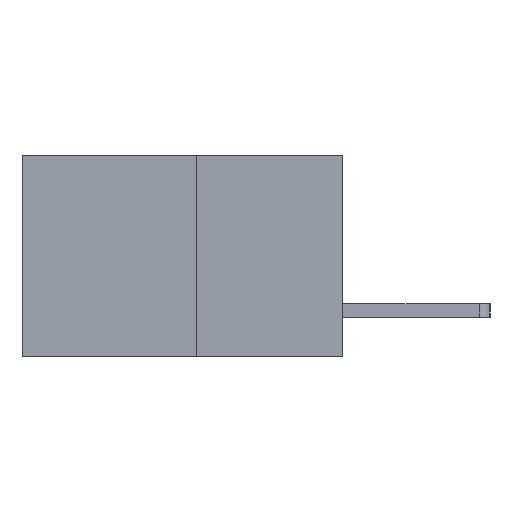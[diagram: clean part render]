
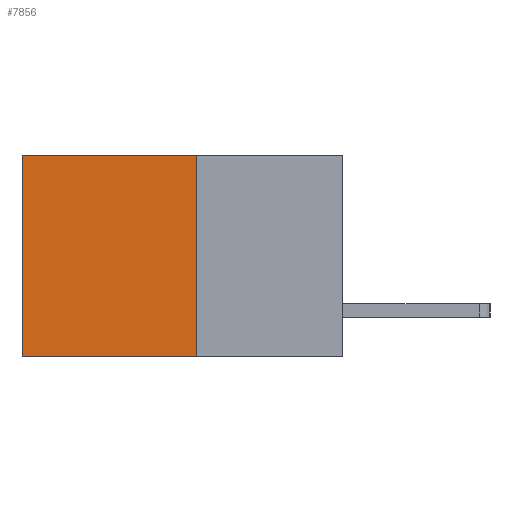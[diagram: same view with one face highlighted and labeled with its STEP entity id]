
A CAD part, left-side view. The second image highlights one B-rep face of the part: STEP entity #7856.
In plain terms, the highlighted planar face has unit normal (-1, 0, 0).
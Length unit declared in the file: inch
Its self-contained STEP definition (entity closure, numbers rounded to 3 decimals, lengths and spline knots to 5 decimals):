
#74 = VECTOR ( 'NONE', #4439, 39.37008 ) ;
#802 = ORIENTED_EDGE ( 'NONE', *, *, #6061, .F. ) ;
#894 = EDGE_LOOP ( 'NONE', ( #6322, #6533, #802, #6768 ) ) ;
#1026 = LINE ( 'NONE', #3760, #4326 ) ;
#1093 = EDGE_CURVE ( 'NONE', #3980, #3262, #3816, .T. ) ;
#1616 = FACE_OUTER_BOUND ( 'NONE', #894, .T. ) ;
#2114 = EDGE_CURVE ( 'NONE', #9240, #6102, #4119, .T. ) ;
#3003 = DIRECTION ( 'NONE',  ( 1., 0., 0. ) ) ;
#3241 = CARTESIAN_POINT ( 'NONE',  ( 0.277, 0.59, -0.37 ) ) ;
#3262 = VERTEX_POINT ( 'NONE', #6713 ) ;
#3725 = VECTOR ( 'NONE', #9517, 39.37008 ) ;
#3760 = CARTESIAN_POINT ( 'NONE',  ( 0.277, 0.27, -0.37 ) ) ;
#3816 = LINE ( 'NONE', #6958, #5563 ) ;
#3980 = VERTEX_POINT ( 'NONE', #6841 ) ;
#4119 = LINE ( 'NONE', #4182, #74 ) ;
#4182 = CARTESIAN_POINT ( 'NONE',  ( 0.277, 0.27, -0.37 ) ) ;
#4271 = AXIS2_PLACEMENT_3D ( 'NONE', #5838, #3003, #9236 ) ;
#4326 = VECTOR ( 'NONE', #6855, 39.37008 ) ;
#4439 = DIRECTION ( 'NONE',  ( 0., 1., 0. ) ) ;
#5562 = DIRECTION ( 'NONE',  ( 0., 1., 0. ) ) ;
#5563 = VECTOR ( 'NONE', #5562, 39.37008 ) ;
#5705 = LINE ( 'NONE', #8768, #3725 ) ;
#5838 = CARTESIAN_POINT ( 'NONE',  ( 0.277, 0.27, -0.37 ) ) ;
#6061 = EDGE_CURVE ( 'NONE', #3980, #9240, #1026, .T. ) ;
#6102 = VERTEX_POINT ( 'NONE', #3241 ) ;
#6322 = ORIENTED_EDGE ( 'NONE', *, *, #9192, .T. ) ;
#6533 = ORIENTED_EDGE ( 'NONE', *, *, #2114, .F. ) ;
#6713 = CARTESIAN_POINT ( 'NONE',  ( 0.277, 0.59, 0. ) ) ;
#6768 = ORIENTED_EDGE ( 'NONE', *, *, #1093, .T. ) ;
#6841 = CARTESIAN_POINT ( 'NONE',  ( 0.277, 0.27, 0. ) ) ;
#6855 = DIRECTION ( 'NONE',  ( 0., 0., -1. ) ) ;
#6958 = CARTESIAN_POINT ( 'NONE',  ( 0.277, 0.27, 0. ) ) ;
#7400 = CARTESIAN_POINT ( 'NONE',  ( 0.277, 0.27, -0.37 ) ) ;
#7802 = PLANE ( 'NONE',  #4271 ) ;
#7856 = ADVANCED_FACE ( 'NONE', ( #1616 ), #7802, .F. ) ;
#8768 = CARTESIAN_POINT ( 'NONE',  ( 0.277, 0.59, -0.37 ) ) ;
#9192 = EDGE_CURVE ( 'NONE', #3262, #6102, #5705, .T. ) ;
#9236 = DIRECTION ( 'NONE',  ( 0., 0., -1. ) ) ;
#9240 = VERTEX_POINT ( 'NONE', #7400 ) ;
#9517 = DIRECTION ( 'NONE',  ( 0., 0., -1. ) ) ;
